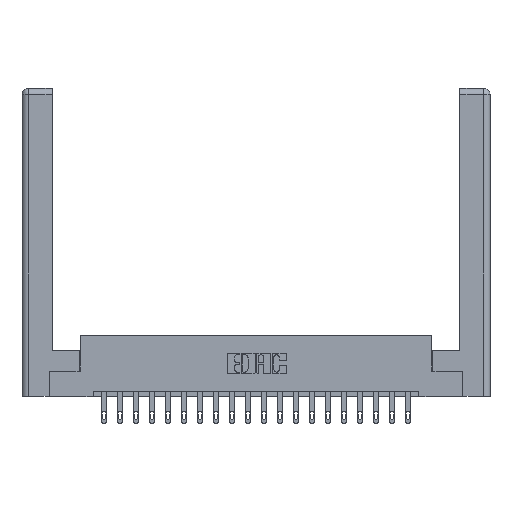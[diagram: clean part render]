
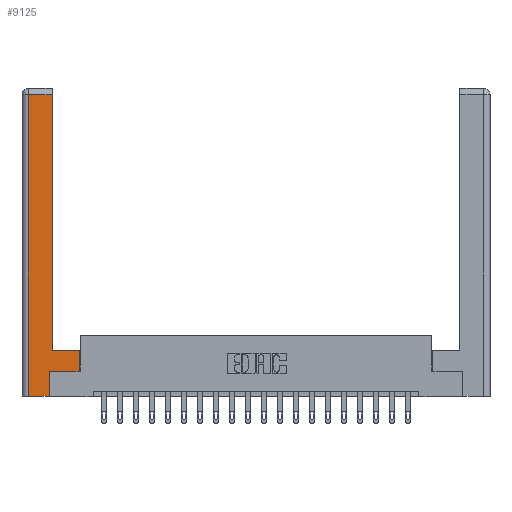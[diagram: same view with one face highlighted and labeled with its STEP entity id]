
A CAD part, top view. The second image highlights one B-rep face of the part: STEP entity #9125.
In plain terms, the highlighted planar face has unit normal (0, 0, 1).
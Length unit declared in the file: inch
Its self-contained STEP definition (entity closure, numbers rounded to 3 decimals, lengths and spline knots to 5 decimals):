
#422 = DIRECTION ( 'NONE',  ( -1., 0., 0. ) ) ;
#508 = CARTESIAN_POINT ( 'NONE',  ( 0.265, 0., 0. ) ) ;
#774 = CARTESIAN_POINT ( 'NONE',  ( 0.295, 2.94, 0. ) ) ;
#798 = CARTESIAN_POINT ( 'NONE',  ( 0.0615, 0., 0. ) ) ;
#1193 = LINE ( 'NONE', #19221, #17415 ) ;
#1614 = ORIENTED_EDGE ( 'NONE', *, *, #5418, .T. ) ;
#1887 = VECTOR ( 'NONE', #13404, 39.37008 ) ;
#2212 = VECTOR ( 'NONE', #19667, 39.37008 ) ;
#2507 = LINE ( 'NONE', #13181, #3780 ) ;
#2558 = VERTEX_POINT ( 'NONE', #3239 ) ;
#2763 = LINE ( 'NONE', #15567, #10352 ) ;
#3219 = ORIENTED_EDGE ( 'NONE', *, *, #5102, .T. ) ;
#3239 = CARTESIAN_POINT ( 'NONE',  ( 0.565, 0.45, 0. ) ) ;
#3755 = DIRECTION ( 'NONE',  ( 0., -1., 0. ) ) ;
#3780 = VECTOR ( 'NONE', #6530, 39.37008 ) ;
#4298 = DIRECTION ( 'NONE',  ( 0., 1., 0. ) ) ;
#4724 = ORIENTED_EDGE ( 'NONE', *, *, #13910, .T. ) ;
#4955 = VECTOR ( 'NONE', #3755, 39.37008 ) ;
#5102 = EDGE_CURVE ( 'NONE', #6896, #7156, #16458, .T. ) ;
#5164 = ORIENTED_EDGE ( 'NONE', *, *, #10898, .T. ) ;
#5418 = EDGE_CURVE ( 'NONE', #20392, #6432, #2763, .T. ) ;
#6154 = CARTESIAN_POINT ( 'NONE',  ( 0.265, 0.245, 0. ) ) ;
#6385 = EDGE_CURVE ( 'NONE', #9520, #6896, #13098, .T. ) ;
#6432 = VERTEX_POINT ( 'NONE', #774 ) ;
#6530 = DIRECTION ( 'NONE',  ( -1., 0., 0. ) ) ;
#6896 = VERTEX_POINT ( 'NONE', #6154 ) ;
#7156 = VERTEX_POINT ( 'NONE', #18476 ) ;
#7898 = CARTESIAN_POINT ( 'NONE',  ( 0., 0., 0. ) ) ;
#9125 = ADVANCED_FACE ( 'NONE', ( #20084 ), #16352, .F. ) ;
#9271 = LINE ( 'NONE', #11898, #4955 ) ;
#9520 = VERTEX_POINT ( 'NONE', #508 ) ;
#9674 = DIRECTION ( 'NONE',  ( 0., 0., -1. ) ) ;
#10352 = VECTOR ( 'NONE', #4298, 39.37008 ) ;
#10387 = VERTEX_POINT ( 'NONE', #17398 ) ;
#10873 = DIRECTION ( 'NONE',  ( 0., 1., 0. ) ) ;
#10898 = EDGE_CURVE ( 'NONE', #2558, #20392, #2507, .T. ) ;
#11638 = CARTESIAN_POINT ( 'NONE',  ( 0.265, 0., 0. ) ) ;
#11898 = CARTESIAN_POINT ( 'NONE',  ( 0.0615, 0., 0. ) ) ;
#12012 = ORIENTED_EDGE ( 'NONE', *, *, #14108, .T. ) ;
#12553 = EDGE_CURVE ( 'NONE', #6432, #10387, #1193, .T. ) ;
#12969 = CARTESIAN_POINT ( 'NONE',  ( 0.565, 0.245, 0. ) ) ;
#13098 = LINE ( 'NONE', #18122, #2212 ) ;
#13117 = EDGE_LOOP ( 'NONE', ( #1614, #16541, #20523, #12012, #13252, #3219, #4724, #5164 ) ) ;
#13181 = CARTESIAN_POINT ( 'NONE',  ( 0.295, 0.45, 0. ) ) ;
#13252 = ORIENTED_EDGE ( 'NONE', *, *, #6385, .T. ) ;
#13404 = DIRECTION ( 'NONE',  ( 1., 0., 0. ) ) ;
#13624 = EDGE_CURVE ( 'NONE', #10387, #18400, #9271, .T. ) ;
#13910 = EDGE_CURVE ( 'NONE', #7156, #2558, #20901, .T. ) ;
#14108 = EDGE_CURVE ( 'NONE', #18400, #9520, #15066, .T. ) ;
#14597 = DIRECTION ( 'NONE',  ( 1., 0., 0. ) ) ;
#14676 = AXIS2_PLACEMENT_3D ( 'NONE', #7898, #9674, #422 ) ;
#15066 = LINE ( 'NONE', #11638, #1887 ) ;
#15567 = CARTESIAN_POINT ( 'NONE',  ( 0.295, 3., 0. ) ) ;
#15969 = DIRECTION ( 'NONE',  ( -1., 0., 0. ) ) ;
#16352 = PLANE ( 'NONE',  #14676 ) ;
#16458 = LINE ( 'NONE', #12969, #17991 ) ;
#16541 = ORIENTED_EDGE ( 'NONE', *, *, #12553, .T. ) ;
#17398 = CARTESIAN_POINT ( 'NONE',  ( 0.0615, 2.94, 0. ) ) ;
#17415 = VECTOR ( 'NONE', #15969, 39.37008 ) ;
#17430 = CARTESIAN_POINT ( 'NONE',  ( 0.565, 0.45, 0. ) ) ;
#17887 = VECTOR ( 'NONE', #10873, 39.37008 ) ;
#17991 = VECTOR ( 'NONE', #14597, 39.37008 ) ;
#18122 = CARTESIAN_POINT ( 'NONE',  ( 0.265, 0.245, 0. ) ) ;
#18400 = VERTEX_POINT ( 'NONE', #798 ) ;
#18476 = CARTESIAN_POINT ( 'NONE',  ( 0.565, 0.245, 0. ) ) ;
#18829 = CARTESIAN_POINT ( 'NONE',  ( 0.295, 0.45, 0. ) ) ;
#19221 = CARTESIAN_POINT ( 'NONE',  ( 0.0615, 2.94, 0. ) ) ;
#19667 = DIRECTION ( 'NONE',  ( 0., 1., 0. ) ) ;
#20084 = FACE_OUTER_BOUND ( 'NONE', #13117, .T. ) ;
#20392 = VERTEX_POINT ( 'NONE', #18829 ) ;
#20523 = ORIENTED_EDGE ( 'NONE', *, *, #13624, .T. ) ;
#20901 = LINE ( 'NONE', #17430, #17887 ) ;
